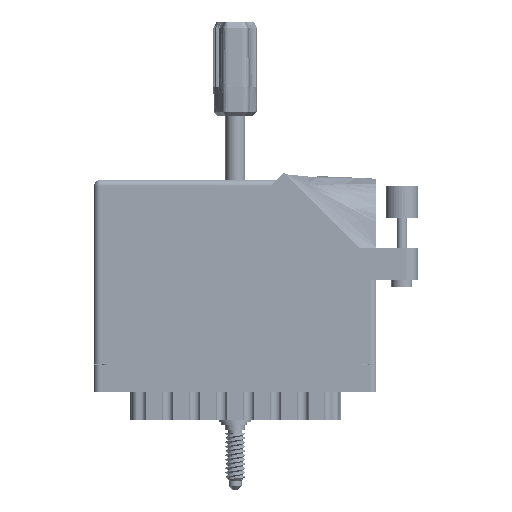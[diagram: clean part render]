
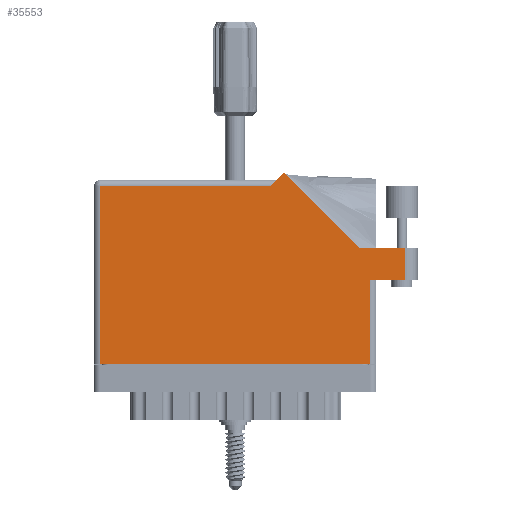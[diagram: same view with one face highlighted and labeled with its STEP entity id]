
A CAD part, front view. The second image highlights one B-rep face of the part: STEP entity #35553.
In plain terms, the highlighted face is planar.
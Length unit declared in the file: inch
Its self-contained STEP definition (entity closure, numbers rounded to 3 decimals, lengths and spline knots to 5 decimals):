
#171 = VECTOR ( 'NONE', #77744, 39.37008 ) ;
#499 = ORIENTED_EDGE ( 'NONE', *, *, #71964, .T. ) ;
#805 = ORIENTED_EDGE ( 'NONE', *, *, #87530, .T. ) ;
#2710 = DIRECTION ( 'NONE',  ( -0.707, -0.707, 0. ) ) ;
#3751 = CARTESIAN_POINT ( 'NONE',  ( 2.993, 1.122, 0. ) ) ;
#4105 = DIRECTION ( 'NONE',  ( -0.707, 0.707, 0. ) ) ;
#8217 = EDGE_CURVE ( 'NONE', #82869, #58824, #70476, .T. ) ;
#13133 = FACE_OUTER_BOUND ( 'NONE', #43809, .T. ) ;
#16729 = DIRECTION ( 'NONE',  ( -1., 0., 0. ) ) ;
#16821 = AXIS2_PLACEMENT_3D ( 'NONE', #40367, #82309, #40941 ) ;
#17276 = VERTEX_POINT ( 'NONE', #41078 ) ;
#18413 = CARTESIAN_POINT ( 'NONE',  ( 2.718, 0.815, 0. ) ) ;
#19929 = ORIENTED_EDGE ( 'NONE', *, *, #49579, .T. ) ;
#20968 = VECTOR ( 'NONE', #2710, 39.37008 ) ;
#22297 = CARTESIAN_POINT ( 'NONE',  ( 1.82871, 1.84571, 0. ) ) ;
#23304 = LINE ( 'NONE', #73279, #57868 ) ;
#26887 = DIRECTION ( 'NONE',  ( 0., 1., 0. ) ) ;
#27253 = CARTESIAN_POINT ( 'NONE',  ( 2.55242, 1.122, 0. ) ) ;
#28361 = VECTOR ( 'NONE', #80021, 39.37008 ) ;
#28445 = LINE ( 'NONE', #68271, #53365 ) ;
#30460 = VERTEX_POINT ( 'NONE', #64948 ) ;
#33157 = ORIENTED_EDGE ( 'NONE', *, *, #52351, .T. ) ;
#33988 = VECTOR ( 'NONE', #4105, 39.37008 ) ;
#35553 = ADVANCED_FACE ( 'NONE', ( #13133 ), #47022, .F. ) ;
#37185 = ORIENTED_EDGE ( 'NONE', *, *, #47434, .T. ) ;
#39212 = DIRECTION ( 'NONE',  ( 1., 0., 0. ) ) ;
#40170 = VERTEX_POINT ( 'NONE', #27253 ) ;
#40180 = CARTESIAN_POINT ( 'NONE',  ( 3.118, 1.122, 0. ) ) ;
#40367 = CARTESIAN_POINT ( 'NONE',  ( 0., 1.775, 0. ) ) ;
#40610 = CARTESIAN_POINT ( 'NONE',  ( 2.656, 0., 0. ) ) ;
#40941 = DIRECTION ( 'NONE',  ( -1., 0., 0. ) ) ;
#41078 = CARTESIAN_POINT ( 'NONE',  ( 0.062, 1.713, 0. ) ) ;
#42726 = VECTOR ( 'NONE', #73418, 39.37008 ) ;
#43021 = LINE ( 'NONE', #18413, #72234 ) ;
#43607 = LINE ( 'NONE', #58368, #75988 ) ;
#43809 = EDGE_LOOP ( 'NONE', ( #19929, #74350, #83319, #805, #37185, #45243, #33157, #44937, #499 ) ) ;
#44937 = ORIENTED_EDGE ( 'NONE', *, *, #8217, .T. ) ;
#45243 = ORIENTED_EDGE ( 'NONE', *, *, #82594, .T. ) ;
#46105 = VERTEX_POINT ( 'NONE', #3751 ) ;
#46270 = CARTESIAN_POINT ( 'NONE',  ( 2.993, 0.815, 0. ) ) ;
#47022 = PLANE ( 'NONE',  #16821 ) ;
#47305 = VERTEX_POINT ( 'NONE', #22297 ) ;
#47434 = EDGE_CURVE ( 'NONE', #47305, #50554, #89051, .T. ) ;
#49579 = EDGE_CURVE ( 'NONE', #30460, #82792, #43021, .T. ) ;
#49783 = CARTESIAN_POINT ( 'NONE',  ( 1.758, 1.775, 0. ) ) ;
#50279 = CARTESIAN_POINT ( 'NONE',  ( 2.656, 0.815, 0. ) ) ;
#50554 = VERTEX_POINT ( 'NONE', #51161 ) ;
#51161 = CARTESIAN_POINT ( 'NONE',  ( 1.696, 1.713, 0. ) ) ;
#52351 = EDGE_CURVE ( 'NONE', #17276, #82869, #23304, .T. ) ;
#52414 = LINE ( 'NONE', #86475, #33988 ) ;
#53365 = VECTOR ( 'NONE', #26887, 39.37008 ) ;
#54399 = CARTESIAN_POINT ( 'NONE',  ( 0.062, 0., 0. ) ) ;
#57868 = VECTOR ( 'NONE', #72690, 39.37008 ) ;
#58368 = CARTESIAN_POINT ( 'NONE',  ( 0., 1.713, 0. ) ) ;
#58824 = VERTEX_POINT ( 'NONE', #40610 ) ;
#63256 = LINE ( 'NONE', #40180, #42726 ) ;
#64948 = CARTESIAN_POINT ( 'NONE',  ( 2.656, 0.815, 0. ) ) ;
#67061 = CARTESIAN_POINT ( 'NONE',  ( 0., 0., 0. ) ) ;
#68271 = CARTESIAN_POINT ( 'NONE',  ( 2.993, 1.122, 0. ) ) ;
#70476 = LINE ( 'NONE', #67061, #28361 ) ;
#71964 = EDGE_CURVE ( 'NONE', #58824, #30460, #86568, .T. ) ;
#72234 = VECTOR ( 'NONE', #39212, 39.37008 ) ;
#72690 = DIRECTION ( 'NONE',  ( 0., -1., 0. ) ) ;
#73279 = CARTESIAN_POINT ( 'NONE',  ( 0.062, 0., 0. ) ) ;
#73418 = DIRECTION ( 'NONE',  ( -1., 0., 0. ) ) ;
#74350 = ORIENTED_EDGE ( 'NONE', *, *, #82871, .T. ) ;
#75988 = VECTOR ( 'NONE', #16729, 39.37008 ) ;
#77744 = DIRECTION ( 'NONE',  ( 0., 1., 0. ) ) ;
#80021 = DIRECTION ( 'NONE',  ( 1., 0., 0. ) ) ;
#81698 = EDGE_CURVE ( 'NONE', #46105, #40170, #63256, .T. ) ;
#82309 = DIRECTION ( 'NONE',  ( 0., 0., -1. ) ) ;
#82594 = EDGE_CURVE ( 'NONE', #50554, #17276, #43607, .T. ) ;
#82792 = VERTEX_POINT ( 'NONE', #46270 ) ;
#82869 = VERTEX_POINT ( 'NONE', #54399 ) ;
#82871 = EDGE_CURVE ( 'NONE', #82792, #46105, #28445, .T. ) ;
#83319 = ORIENTED_EDGE ( 'NONE', *, *, #81698, .T. ) ;
#86475 = CARTESIAN_POINT ( 'NONE',  ( 2.55242, 1.122, 0. ) ) ;
#86568 = LINE ( 'NONE', #50279, #171 ) ;
#87530 = EDGE_CURVE ( 'NONE', #40170, #47305, #52414, .T. ) ;
#89051 = LINE ( 'NONE', #49783, #20968 ) ;
